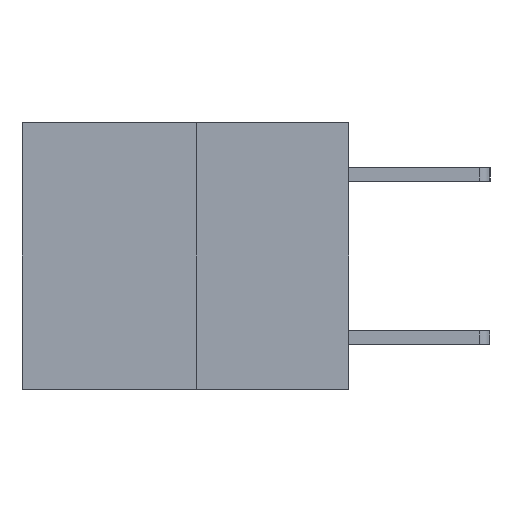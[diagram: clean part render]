
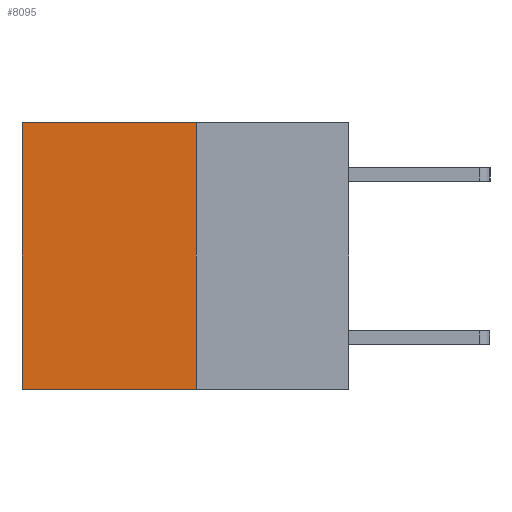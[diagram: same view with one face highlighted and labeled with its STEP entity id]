
A CAD part, left-side view. The second image highlights one B-rep face of the part: STEP entity #8095.
In plain terms, the highlighted planar face has unit normal (-1, 0, 0).
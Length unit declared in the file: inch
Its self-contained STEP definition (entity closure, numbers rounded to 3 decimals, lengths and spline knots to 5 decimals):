
#339 = ORIENTED_EDGE ( 'NONE', *, *, #1150, .F. ) ;
#379 = VERTEX_POINT ( 'NONE', #6003 ) ;
#616 = CARTESIAN_POINT ( 'NONE',  ( 0.3165, 0.28, 0. ) ) ;
#891 = CARTESIAN_POINT ( 'NONE',  ( 0.3165, 0.28, -0.49 ) ) ;
#980 = CARTESIAN_POINT ( 'NONE',  ( 0.3165, 0.6, 0. ) ) ;
#1150 = EDGE_CURVE ( 'NONE', #2455, #379, #3266, .T. ) ;
#1187 = DIRECTION ( 'NONE',  ( 0., 0., -1. ) ) ;
#1396 = DIRECTION ( 'NONE',  ( 0., 1., 0. ) ) ;
#1906 = DIRECTION ( 'NONE',  ( 1., 0., 0. ) ) ;
#1910 = CARTESIAN_POINT ( 'NONE',  ( 0.3165, 0.28, -0.49 ) ) ;
#1982 = ORIENTED_EDGE ( 'NONE', *, *, #2050, .T. ) ;
#2050 = EDGE_CURVE ( 'NONE', #5680, #8142, #5196, .T. ) ;
#2080 = CARTESIAN_POINT ( 'NONE',  ( 0.3165, 0.6, -0.49 ) ) ;
#2103 = CARTESIAN_POINT ( 'NONE',  ( 0.3165, 0.28, 0. ) ) ;
#2392 = LINE ( 'NONE', #1910, #4977 ) ;
#2455 = VERTEX_POINT ( 'NONE', #891 ) ;
#2851 = VECTOR ( 'NONE', #1396, 39.37008 ) ;
#2860 = LINE ( 'NONE', #2080, #8610 ) ;
#2922 = FACE_OUTER_BOUND ( 'NONE', #5706, .T. ) ;
#2942 = AXIS2_PLACEMENT_3D ( 'NONE', #5869, #1906, #1187 ) ;
#3266 = LINE ( 'NONE', #4765, #2851 ) ;
#4744 = EDGE_CURVE ( 'NONE', #8142, #379, #2860, .T. ) ;
#4765 = CARTESIAN_POINT ( 'NONE',  ( 0.3165, 0.28, -0.49 ) ) ;
#4977 = VECTOR ( 'NONE', #8845, 39.37008 ) ;
#5196 = LINE ( 'NONE', #2103, #5767 ) ;
#5680 = VERTEX_POINT ( 'NONE', #616 ) ;
#5706 = EDGE_LOOP ( 'NONE', ( #8066, #339, #7662, #1982 ) ) ;
#5767 = VECTOR ( 'NONE', #6245, 39.37008 ) ;
#5869 = CARTESIAN_POINT ( 'NONE',  ( 0.3165, 0.28, -0.49 ) ) ;
#6003 = CARTESIAN_POINT ( 'NONE',  ( 0.3165, 0.6, -0.49 ) ) ;
#6245 = DIRECTION ( 'NONE',  ( 0., 1., 0. ) ) ;
#6782 = PLANE ( 'NONE',  #2942 ) ;
#7630 = DIRECTION ( 'NONE',  ( 0., 0., -1. ) ) ;
#7662 = ORIENTED_EDGE ( 'NONE', *, *, #8638, .F. ) ;
#8066 = ORIENTED_EDGE ( 'NONE', *, *, #4744, .T. ) ;
#8095 = ADVANCED_FACE ( 'NONE', ( #2922 ), #6782, .F. ) ;
#8142 = VERTEX_POINT ( 'NONE', #980 ) ;
#8610 = VECTOR ( 'NONE', #7630, 39.37008 ) ;
#8638 = EDGE_CURVE ( 'NONE', #5680, #2455, #2392, .T. ) ;
#8845 = DIRECTION ( 'NONE',  ( 0., 0., -1. ) ) ;
